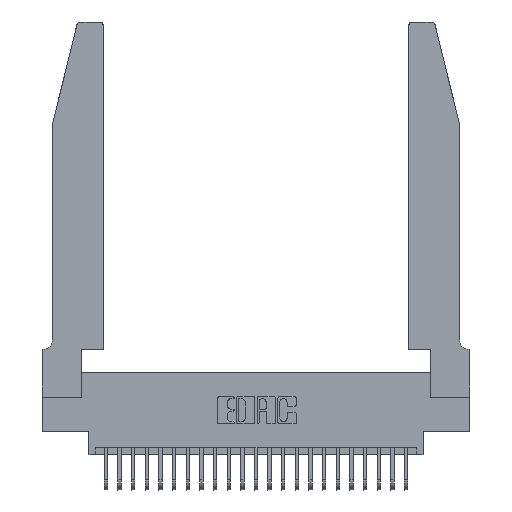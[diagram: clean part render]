
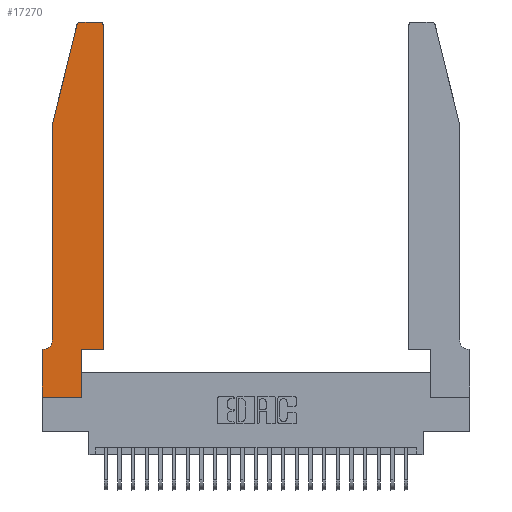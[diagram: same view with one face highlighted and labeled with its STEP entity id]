
A CAD part, top view. The second image highlights one B-rep face of the part: STEP entity #17270.
In plain terms, the highlighted planar face has unit normal (0, 0, 1).
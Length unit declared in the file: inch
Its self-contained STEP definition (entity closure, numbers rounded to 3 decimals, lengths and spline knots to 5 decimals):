
#401 = VERTEX_POINT ( 'NONE', #25033 ) ;
#1102 = VECTOR ( 'NONE', #17949, 39.37008 ) ;
#1465 = VECTOR ( 'NONE', #26686, 39.37008 ) ;
#1782 = CARTESIAN_POINT ( 'NONE',  ( 0., 0.35, 0.37 ) ) ;
#1876 = CARTESIAN_POINT ( 'NONE',  ( 0.0755, 2., 0.37 ) ) ;
#1896 = DIRECTION ( 'NONE',  ( 0., -1., 0. ) ) ;
#2117 = ORIENTED_EDGE ( 'NONE', *, *, #21283, .T. ) ;
#2221 = CARTESIAN_POINT ( 'NONE',  ( 0.0755, 0.42, 0.37 ) ) ;
#2288 = ORIENTED_EDGE ( 'NONE', *, *, #5716, .T. ) ;
#2464 = CARTESIAN_POINT ( 'NONE',  ( 0.0755, 2., 0.37 ) ) ;
#2935 = CARTESIAN_POINT ( 'NONE',  ( 0.4205, 2.72, 0.37 ) ) ;
#3144 = CARTESIAN_POINT ( 'NONE',  ( 0.4505, 0.35, 0.37 ) ) ;
#3202 = CARTESIAN_POINT ( 'NONE',  ( 0., 0., 0.37 ) ) ;
#3714 = CIRCLE ( 'NONE', #23128, 0.03 ) ;
#3888 = DIRECTION ( 'NONE',  ( 1., 0., 0. ) ) ;
#4523 = CARTESIAN_POINT ( 'NONE',  ( 0.284, 2.72, 0.37 ) ) ;
#4863 = VERTEX_POINT ( 'NONE', #2221 ) ;
#5032 = DIRECTION ( 'NONE',  ( 1., 0., 0. ) ) ;
#5352 = DIRECTION ( 'NONE',  ( 1., 0., 0. ) ) ;
#5647 = CARTESIAN_POINT ( 'NONE',  ( 0.0055, 0.42, 0.37 ) ) ;
#5716 = EDGE_CURVE ( 'NONE', #14326, #26343, #22785, .T. ) ;
#5946 = EDGE_CURVE ( 'NONE', #18066, #4863, #23765, .T. ) ;
#5999 = LINE ( 'NONE', #1876, #12302 ) ;
#6622 = DIRECTION ( 'NONE',  ( 1., 0., 0. ) ) ;
#6954 = ORIENTED_EDGE ( 'NONE', *, *, #25856, .T. ) ;
#7314 = CARTESIAN_POINT ( 'NONE',  ( 0.25487, 2.72718, 0.37 ) ) ;
#7595 = CARTESIAN_POINT ( 'NONE',  ( 0.2865, 0.35, 0.37 ) ) ;
#7674 = LINE ( 'NONE', #12067, #1465 ) ;
#7717 = DIRECTION ( 'NONE',  ( 0., 1., 0. ) ) ;
#7729 = DIRECTION ( 'NONE',  ( -1., 0., 0. ) ) ;
#7763 = VERTEX_POINT ( 'NONE', #8700 ) ;
#7937 = EDGE_CURVE ( 'NONE', #17109, #27017, #3714, .T. ) ;
#8700 = CARTESIAN_POINT ( 'NONE',  ( 0.284, 2.75, 0.37 ) ) ;
#8803 = EDGE_CURVE ( 'NONE', #20269, #18066, #5999, .T. ) ;
#8874 = VECTOR ( 'NONE', #13238, 39.37008 ) ;
#9068 = CARTESIAN_POINT ( 'NONE',  ( 0.4505, 0.35, 0.37 ) ) ;
#9139 = EDGE_CURVE ( 'NONE', #26440, #10706, #26016, .T. ) ;
#9246 = ORIENTED_EDGE ( 'NONE', *, *, #9139, .T. ) ;
#9737 = LINE ( 'NONE', #26466, #25165 ) ;
#10021 = DIRECTION ( 'NONE',  ( -1., 0., 0. ) ) ;
#10706 = VERTEX_POINT ( 'NONE', #9068 ) ;
#10794 = CARTESIAN_POINT ( 'NONE',  ( 0., 0.35, 0.37 ) ) ;
#11049 = ORIENTED_EDGE ( 'NONE', *, *, #20962, .T. ) ;
#11654 = ORIENTED_EDGE ( 'NONE', *, *, #8803, .T. ) ;
#12067 = CARTESIAN_POINT ( 'NONE',  ( 0., 0., 0.37 ) ) ;
#12132 = AXIS2_PLACEMENT_3D ( 'NONE', #4523, #19263, #6622 ) ;
#12302 = VECTOR ( 'NONE', #14508, 39.37008 ) ;
#13109 = ORIENTED_EDGE ( 'NONE', *, *, #15941, .T. ) ;
#13238 = DIRECTION ( 'NONE',  ( 0., 1., 0. ) ) ;
#13471 = EDGE_CURVE ( 'NONE', #26343, #401, #7674, .T. ) ;
#13571 = CARTESIAN_POINT ( 'NONE',  ( 0., 0., 0.37 ) ) ;
#13966 = CARTESIAN_POINT ( 'NONE',  ( 0.4505, 2.72, 0.37 ) ) ;
#14029 = AXIS2_PLACEMENT_3D ( 'NONE', #1782, #16552, #3888 ) ;
#14079 = AXIS2_PLACEMENT_3D ( 'NONE', #5647, #20367, #7729 ) ;
#14326 = VERTEX_POINT ( 'NONE', #10794 ) ;
#14508 = DIRECTION ( 'NONE',  ( -0.239, -0.971, 0. ) ) ;
#14944 = VERTEX_POINT ( 'NONE', #22955 ) ;
#15530 = VECTOR ( 'NONE', #10021, 39.37008 ) ;
#15744 = EDGE_CURVE ( 'NONE', #10706, #17109, #17175, .T. ) ;
#15941 = EDGE_CURVE ( 'NONE', #14944, #14326, #21035, .T. ) ;
#16446 = VECTOR ( 'NONE', #7717, 39.37008 ) ;
#16536 = ORIENTED_EDGE ( 'NONE', *, *, #19117, .T. ) ;
#16552 = DIRECTION ( 'NONE',  ( 0., 0., 1. ) ) ;
#17109 = VERTEX_POINT ( 'NONE', #13966 ) ;
#17175 = LINE ( 'NONE', #19561, #8874 ) ;
#17270 = ADVANCED_FACE ( 'NONE', ( #23593 ), #18542, .T. ) ;
#17573 = VECTOR ( 'NONE', #1896, 39.37008 ) ;
#17668 = DIRECTION ( 'NONE',  ( 0., 0., 1. ) ) ;
#17949 = DIRECTION ( 'NONE',  ( 0., -1., 0. ) ) ;
#18066 = VERTEX_POINT ( 'NONE', #2464 ) ;
#18296 = CIRCLE ( 'NONE', #14079, 0.07 ) ;
#18542 = PLANE ( 'NONE',  #14029 ) ;
#18621 = EDGE_LOOP ( 'NONE', ( #16536, #2117, #11654, #19599, #11049, #13109, #2288, #19238, #6954, #9246, #21993, #24934 ) ) ;
#19117 = EDGE_CURVE ( 'NONE', #27017, #7763, #9737, .T. ) ;
#19238 = ORIENTED_EDGE ( 'NONE', *, *, #13471, .T. ) ;
#19263 = DIRECTION ( 'NONE',  ( 0., 0., 1. ) ) ;
#19561 = CARTESIAN_POINT ( 'NONE',  ( 0.4505, 0.35, 0.37 ) ) ;
#19599 = ORIENTED_EDGE ( 'NONE', *, *, #5946, .T. ) ;
#19825 = VECTOR ( 'NONE', #5352, 39.37008 ) ;
#20269 = VERTEX_POINT ( 'NONE', #7314 ) ;
#20367 = DIRECTION ( 'NONE',  ( 0., 0., -1. ) ) ;
#20593 = CARTESIAN_POINT ( 'NONE',  ( 0.0755, 0.35, 0.37 ) ) ;
#20962 = EDGE_CURVE ( 'NONE', #4863, #14944, #18296, .T. ) ;
#21035 = LINE ( 'NONE', #20593, #15530 ) ;
#21283 = EDGE_CURVE ( 'NONE', #7763, #20269, #21509, .T. ) ;
#21509 = CIRCLE ( 'NONE', #12132, 0.03 ) ;
#21950 = LINE ( 'NONE', #24453, #16446 ) ;
#21993 = ORIENTED_EDGE ( 'NONE', *, *, #15744, .T. ) ;
#22270 = DIRECTION ( 'NONE',  ( -1., 0., 0. ) ) ;
#22785 = LINE ( 'NONE', #3202, #1102 ) ;
#22955 = CARTESIAN_POINT ( 'NONE',  ( 0.0055, 0.35, 0.37 ) ) ;
#23128 = AXIS2_PLACEMENT_3D ( 'NONE', #2935, #17668, #5032 ) ;
#23593 = FACE_OUTER_BOUND ( 'NONE', #18621, .T. ) ;
#23765 = LINE ( 'NONE', #24935, #17573 ) ;
#24453 = CARTESIAN_POINT ( 'NONE',  ( 0.2865, 0.35, 0.37 ) ) ;
#24934 = ORIENTED_EDGE ( 'NONE', *, *, #7937, .T. ) ;
#24935 = CARTESIAN_POINT ( 'NONE',  ( 0.0755, 2., 0.37 ) ) ;
#25033 = CARTESIAN_POINT ( 'NONE',  ( 0.2865, 0., 0.37 ) ) ;
#25165 = VECTOR ( 'NONE', #22270, 39.37008 ) ;
#25856 = EDGE_CURVE ( 'NONE', #401, #26440, #21950, .T. ) ;
#26016 = LINE ( 'NONE', #3144, #19825 ) ;
#26038 = CARTESIAN_POINT ( 'NONE',  ( 0.4205, 2.75, 0.37 ) ) ;
#26343 = VERTEX_POINT ( 'NONE', #13571 ) ;
#26440 = VERTEX_POINT ( 'NONE', #7595 ) ;
#26466 = CARTESIAN_POINT ( 'NONE',  ( 0.2605, 2.75, 0.37 ) ) ;
#26686 = DIRECTION ( 'NONE',  ( 1., 0., 0. ) ) ;
#27017 = VERTEX_POINT ( 'NONE', #26038 ) ;
